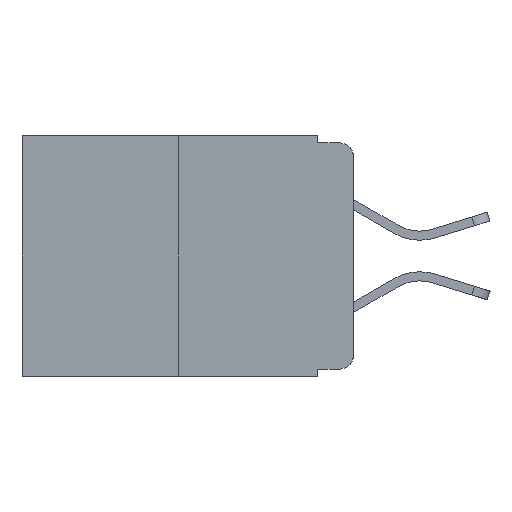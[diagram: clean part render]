
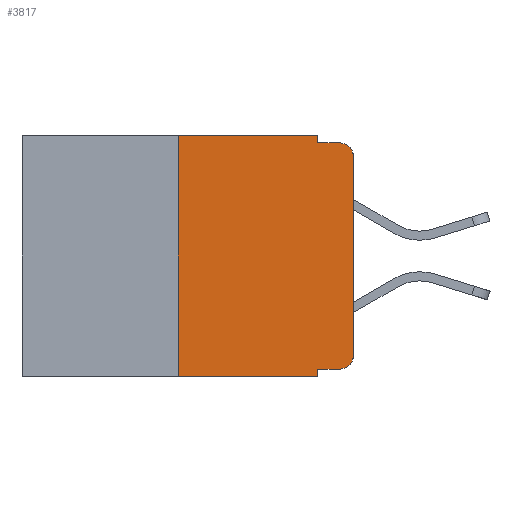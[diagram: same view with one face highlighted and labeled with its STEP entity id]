
A CAD part, left-side view. The second image highlights one B-rep face of the part: STEP entity #3817.
In plain terms, the highlighted planar face has unit normal (-1, 0, 0).
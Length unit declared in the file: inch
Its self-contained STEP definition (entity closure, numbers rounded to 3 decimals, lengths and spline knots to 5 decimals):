
#84 = DIRECTION ( 'NONE',  ( 0., 0., -1. ) ) ;
#175 = LINE ( 'NONE', #3085, #11548 ) ;
#590 = AXIS2_PLACEMENT_3D ( 'NONE', #13738, #8201, #7012 ) ;
#709 = ORIENTED_EDGE ( 'NONE', *, *, #10393, .T. ) ;
#749 = CARTESIAN_POINT ( 'NONE',  ( 0., 0.051, 0. ) ) ;
#782 = EDGE_CURVE ( 'NONE', #13879, #5157, #5914, .T. ) ;
#972 = LINE ( 'NONE', #13218, #7089 ) ;
#993 = ORIENTED_EDGE ( 'NONE', *, *, #5011, .F. ) ;
#1096 = VECTOR ( 'NONE', #5992, 39.37008 ) ;
#1224 = VERTEX_POINT ( 'NONE', #8471 ) ;
#1402 = EDGE_LOOP ( 'NONE', ( #13741, #709, #993, #12008, #8047, #11279, #13250, #7417, #4984, #3169 ) ) ;
#1478 = CARTESIAN_POINT ( 'NONE',  ( 0., 0.473, 0. ) ) ;
#1499 = VERTEX_POINT ( 'NONE', #3435 ) ;
#1524 = LINE ( 'NONE', #10128, #4672 ) ;
#1797 = VECTOR ( 'NONE', #5934, 39.37008 ) ;
#1872 = LINE ( 'NONE', #13451, #11532 ) ;
#2278 = FACE_OUTER_BOUND ( 'NONE', #1402, .T. ) ;
#2861 = AXIS2_PLACEMENT_3D ( 'NONE', #6139, #14100, #7383 ) ;
#3085 = CARTESIAN_POINT ( 'NONE',  ( 0., 0.051, -0.01 ) ) ;
#3169 = ORIENTED_EDGE ( 'NONE', *, *, #8637, .T. ) ;
#3246 = CARTESIAN_POINT ( 'NONE',  ( 0., 0.02, -0.333 ) ) ;
#3397 = AXIS2_PLACEMENT_3D ( 'NONE', #7121, #9530, #4921 ) ;
#3435 = CARTESIAN_POINT ( 'NONE',  ( 0., 0.051, -0.01 ) ) ;
#3595 = EDGE_CURVE ( 'NONE', #10462, #1499, #8420, .T. ) ;
#3817 = ADVANCED_FACE ( 'NONE', ( #2278 ), #12858, .F. ) ;
#3918 = CIRCLE ( 'NONE', #590, 0.02 ) ;
#4161 = CARTESIAN_POINT ( 'NONE',  ( 0., 0.473, -0.343 ) ) ;
#4208 = EDGE_CURVE ( 'NONE', #13879, #4529, #11740, .T. ) ;
#4271 = DIRECTION ( 'NONE',  ( 0., -1., 0. ) ) ;
#4529 = VERTEX_POINT ( 'NONE', #11390 ) ;
#4672 = VECTOR ( 'NONE', #5634, 39.37008 ) ;
#4891 = CARTESIAN_POINT ( 'NONE',  ( 0., 0.051, 0. ) ) ;
#4921 = DIRECTION ( 'NONE',  ( 0., 0., -1. ) ) ;
#4984 = ORIENTED_EDGE ( 'NONE', *, *, #6450, .T. ) ;
#5011 = EDGE_CURVE ( 'NONE', #1499, #6404, #175, .T. ) ;
#5157 = VERTEX_POINT ( 'NONE', #6740 ) ;
#5317 = DIRECTION ( 'NONE',  ( 0., -1., 0. ) ) ;
#5634 = DIRECTION ( 'NONE',  ( 0., 0., 1. ) ) ;
#5769 = CARTESIAN_POINT ( 'NONE',  ( 0., 0.25, 0. ) ) ;
#5914 = LINE ( 'NONE', #5769, #1096 ) ;
#5934 = DIRECTION ( 'NONE',  ( 0., -1., 0. ) ) ;
#5992 = DIRECTION ( 'NONE',  ( 0., 0., 1. ) ) ;
#6088 = VERTEX_POINT ( 'NONE', #12330 ) ;
#6139 = CARTESIAN_POINT ( 'NONE',  ( 0., 0.473, 0. ) ) ;
#6340 = CARTESIAN_POINT ( 'NONE',  ( 0., 0.25, -0.343 ) ) ;
#6404 = VERTEX_POINT ( 'NONE', #13313 ) ;
#6450 = EDGE_CURVE ( 'NONE', #9561, #11981, #972, .T. ) ;
#6740 = CARTESIAN_POINT ( 'NONE',  ( 0., 0.25, 0. ) ) ;
#7012 = DIRECTION ( 'NONE',  ( 0., 0., -1. ) ) ;
#7089 = VECTOR ( 'NONE', #4271, 39.37008 ) ;
#7121 = CARTESIAN_POINT ( 'NONE',  ( 0., 0.02, -0.313 ) ) ;
#7383 = DIRECTION ( 'NONE',  ( 0., 0., -1. ) ) ;
#7417 = ORIENTED_EDGE ( 'NONE', *, *, #9172, .F. ) ;
#8015 = EDGE_CURVE ( 'NONE', #5157, #10462, #10057, .T. ) ;
#8047 = ORIENTED_EDGE ( 'NONE', *, *, #8015, .F. ) ;
#8201 = DIRECTION ( 'NONE',  ( -1., 0., 0. ) ) ;
#8420 = LINE ( 'NONE', #4891, #11060 ) ;
#8471 = CARTESIAN_POINT ( 'NONE',  ( 0., 0., -0.313 ) ) ;
#8637 = EDGE_CURVE ( 'NONE', #11981, #1224, #13628, .T. ) ;
#9089 = EDGE_CURVE ( 'NONE', #1224, #6088, #1524, .T. ) ;
#9172 = EDGE_CURVE ( 'NONE', #9561, #4529, #1872, .T. ) ;
#9530 = DIRECTION ( 'NONE',  ( -1., 0., 0. ) ) ;
#9561 = VERTEX_POINT ( 'NONE', #13535 ) ;
#9562 = DIRECTION ( 'NONE',  ( 0., 0., -1. ) ) ;
#10057 = LINE ( 'NONE', #1478, #1797 ) ;
#10128 = CARTESIAN_POINT ( 'NONE',  ( 0., 0., 0. ) ) ;
#10393 = EDGE_CURVE ( 'NONE', #6088, #6404, #3918, .T. ) ;
#10462 = VERTEX_POINT ( 'NONE', #749 ) ;
#11060 = VECTOR ( 'NONE', #84, 39.37008 ) ;
#11279 = ORIENTED_EDGE ( 'NONE', *, *, #782, .F. ) ;
#11390 = CARTESIAN_POINT ( 'NONE',  ( 0., 0.051, -0.343 ) ) ;
#11532 = VECTOR ( 'NONE', #9562, 39.37008 ) ;
#11548 = VECTOR ( 'NONE', #5317, 39.37008 ) ;
#11740 = LINE ( 'NONE', #4161, #13834 ) ;
#11981 = VERTEX_POINT ( 'NONE', #3246 ) ;
#12008 = ORIENTED_EDGE ( 'NONE', *, *, #3595, .F. ) ;
#12330 = CARTESIAN_POINT ( 'NONE',  ( 0., 0., -0.03 ) ) ;
#12858 = PLANE ( 'NONE',  #2861 ) ;
#13218 = CARTESIAN_POINT ( 'NONE',  ( 0., 0.051, -0.333 ) ) ;
#13250 = ORIENTED_EDGE ( 'NONE', *, *, #4208, .T. ) ;
#13313 = CARTESIAN_POINT ( 'NONE',  ( 0., 0.02, -0.01 ) ) ;
#13451 = CARTESIAN_POINT ( 'NONE',  ( 0., 0.051, 0. ) ) ;
#13480 = DIRECTION ( 'NONE',  ( 0., -1., 0. ) ) ;
#13535 = CARTESIAN_POINT ( 'NONE',  ( 0., 0.051, -0.333 ) ) ;
#13628 = CIRCLE ( 'NONE', #3397, 0.02 ) ;
#13738 = CARTESIAN_POINT ( 'NONE',  ( 0., 0.02, -0.03 ) ) ;
#13741 = ORIENTED_EDGE ( 'NONE', *, *, #9089, .T. ) ;
#13834 = VECTOR ( 'NONE', #13480, 39.37008 ) ;
#13879 = VERTEX_POINT ( 'NONE', #6340 ) ;
#14100 = DIRECTION ( 'NONE',  ( 1., 0., 0. ) ) ;
